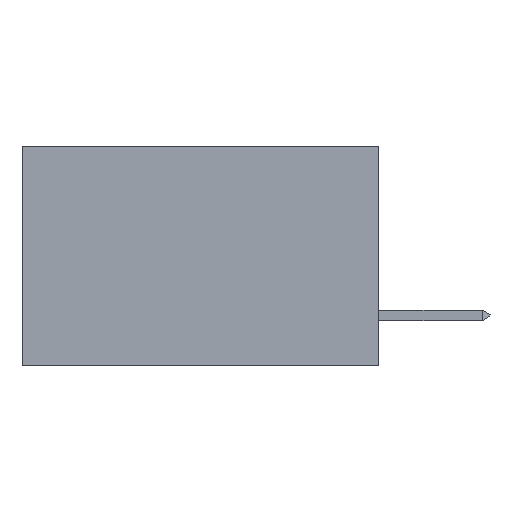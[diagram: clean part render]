
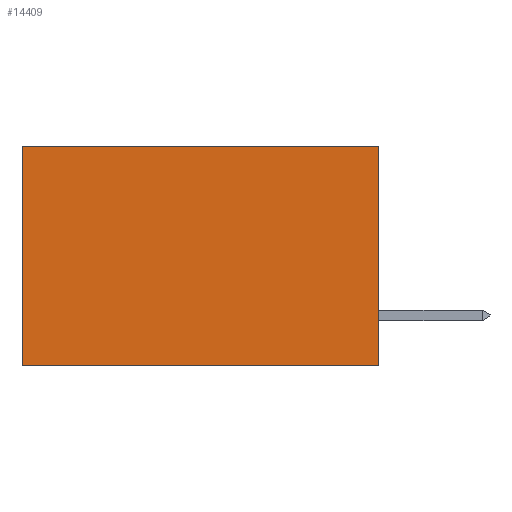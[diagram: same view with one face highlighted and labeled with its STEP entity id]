
A CAD part, left-side view. The second image highlights one B-rep face of the part: STEP entity #14409.
In plain terms, the highlighted planar face has unit normal (-1, 0, 0).
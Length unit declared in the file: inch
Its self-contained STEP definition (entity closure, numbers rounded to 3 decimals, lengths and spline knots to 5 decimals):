
#1949 = EDGE_CURVE ( 'NONE', #5080, #14388, #9193, .T. ) ;
#3526 = CARTESIAN_POINT ( 'NONE',  ( 0.298, 0.6, -0.37 ) ) ;
#4155 = DIRECTION ( 'NONE',  ( 0., 0., -1. ) ) ;
#5080 = VERTEX_POINT ( 'NONE', #13769 ) ;
#7162 = DIRECTION ( 'NONE',  ( 0., 1., 0. ) ) ;
#7338 = CARTESIAN_POINT ( 'NONE',  ( 0.298, 0., -0.37 ) ) ;
#9193 = LINE ( 'NONE', #7338, #16653 ) ;
#9275 = ORIENTED_EDGE ( 'NONE', *, *, #18827, .F. ) ;
#10734 = CARTESIAN_POINT ( 'NONE',  ( 0.298, 0., 0. ) ) ;
#11357 = VECTOR ( 'NONE', #16606, 39.37008 ) ;
#11779 = DIRECTION ( 'NONE',  ( 0., 0., -1. ) ) ;
#11896 = VERTEX_POINT ( 'NONE', #22452 ) ;
#12053 = CARTESIAN_POINT ( 'NONE',  ( 0.298, 0., 0. ) ) ;
#12061 = VERTEX_POINT ( 'NONE', #18270 ) ;
#12229 = DIRECTION ( 'NONE',  ( 1., 0., 0. ) ) ;
#12413 = PLANE ( 'NONE',  #20366 ) ;
#13769 = CARTESIAN_POINT ( 'NONE',  ( 0.298, 0., -0.37 ) ) ;
#14256 = ORIENTED_EDGE ( 'NONE', *, *, #17450, .T. ) ;
#14388 = VERTEX_POINT ( 'NONE', #3526 ) ;
#14409 = ADVANCED_FACE ( 'NONE', ( #21506 ), #12413, .F. ) ;
#14582 = EDGE_CURVE ( 'NONE', #12061, #14388, #18882, .T. ) ;
#15645 = CARTESIAN_POINT ( 'NONE',  ( 0.298, 0.6, 0. ) ) ;
#16606 = DIRECTION ( 'NONE',  ( 0., 1., 0. ) ) ;
#16653 = VECTOR ( 'NONE', #7162, 39.37008 ) ;
#17450 = EDGE_CURVE ( 'NONE', #11896, #12061, #22318, .T. ) ;
#18270 = CARTESIAN_POINT ( 'NONE',  ( 0.298, 0.6, 0. ) ) ;
#18827 = EDGE_CURVE ( 'NONE', #11896, #5080, #24821, .T. ) ;
#18882 = LINE ( 'NONE', #15645, #22771 ) ;
#19653 = VECTOR ( 'NONE', #11779, 39.37008 ) ;
#19951 = ORIENTED_EDGE ( 'NONE', *, *, #1949, .F. ) ;
#20366 = AXIS2_PLACEMENT_3D ( 'NONE', #12053, #12229, #4155 ) ;
#20452 = EDGE_LOOP ( 'NONE', ( #23644, #19951, #9275, #14256 ) ) ;
#21506 = FACE_OUTER_BOUND ( 'NONE', #20452, .T. ) ;
#22318 = LINE ( 'NONE', #10734, #11357 ) ;
#22452 = CARTESIAN_POINT ( 'NONE',  ( 0.298, 0., 0. ) ) ;
#22771 = VECTOR ( 'NONE', #23955, 39.37008 ) ;
#23644 = ORIENTED_EDGE ( 'NONE', *, *, #14582, .T. ) ;
#23955 = DIRECTION ( 'NONE',  ( 0., 0., -1. ) ) ;
#24821 = LINE ( 'NONE', #25565, #19653 ) ;
#25565 = CARTESIAN_POINT ( 'NONE',  ( 0.298, 0., 0. ) ) ;
